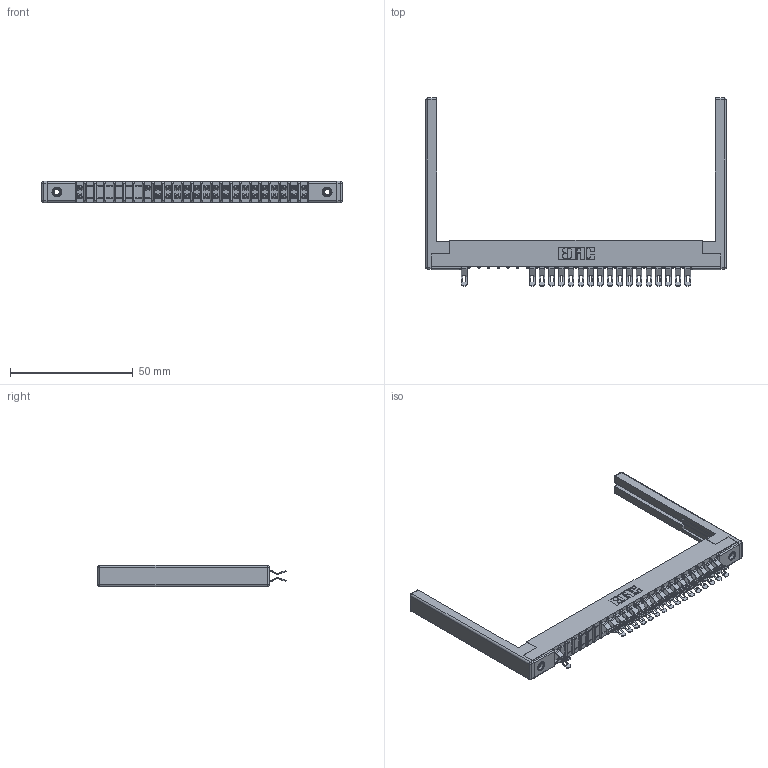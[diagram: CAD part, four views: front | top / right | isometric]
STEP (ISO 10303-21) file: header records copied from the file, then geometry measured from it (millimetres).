
FILE_DESCRIPTION (( 'STEP AP203' ), '1' );
FILE_NAME ('307-048-555-268.STEP', '2018-08-06T03:56:00', ( '' ), ( '' ), 'SwSTEP 2.0', 'SolidWorks 2016', '' );
FILE_SCHEMA (( 'CONFIG_CONTROL_DESIGN' ));
Length unit declared in the file: inch
Products named in the file (5): 345-250-001_345-250-001-102; 307-048-555-268; 307 Part_.156 Dia Mounting Holes; 307-290-001_555; 307-220-068
Assembly tree (40 placements, depth 2):
  307-048-555-268
    307 Part_.156 Dia Mounting Holes
    307-290-001_555  x35
    307-220-068  x2
    345-250-001_345-250-001-102  x2
Bounding box: 122.53 x 76.71 x 8.71 mm (x, y, z)
Volume: 12512 mm3; surface area: 17772.7 mm2
Topology: 40 solids, 40 shells, 2562 faces, 7464 edges, 4840 vertices
Faces by surface type: plane 1426, cylinder 1062, sphere 58, cone 12, torus 4
Entity records: 26442 total; most frequent: CARTESIAN_POINT 4368, ORIENTED_EDGE 4334, DIRECTION 4295, EDGE_CURVE 2167, LINE 1641, VECTOR 1641, VERTEX_POINT 1400, AXIS2_PLACEMENT_3D 1327
